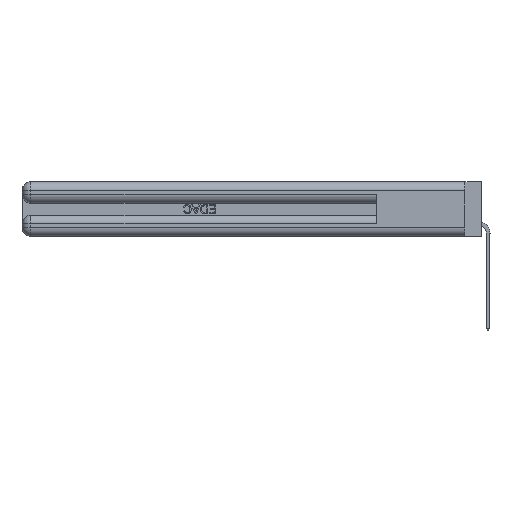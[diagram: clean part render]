
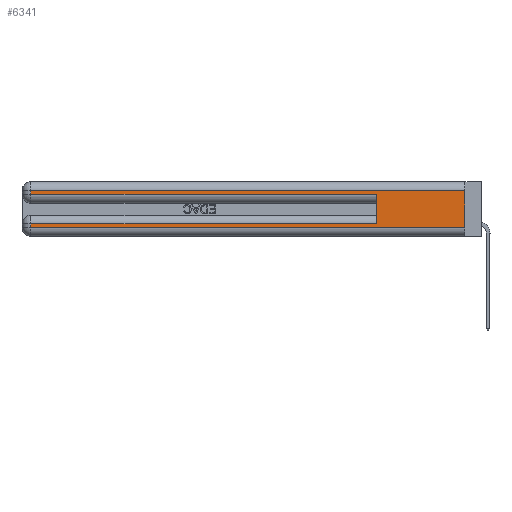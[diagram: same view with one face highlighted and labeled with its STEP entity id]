
A CAD part, left-side view. The second image highlights one B-rep face of the part: STEP entity #6341.
In plain terms, the highlighted planar face has unit normal (-1, 0, 0).
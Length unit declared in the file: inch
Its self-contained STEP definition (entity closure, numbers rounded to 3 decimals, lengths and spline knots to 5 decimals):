
#353 = VECTOR ( 'NONE', #24202, 39.37008 ) ;
#382 = CARTESIAN_POINT ( 'NONE',  ( 0., 0., 0.06 ) ) ;
#565 = EDGE_CURVE ( 'NONE', #36452, #20601, #5713, .T. ) ;
#597 = VECTOR ( 'NONE', #34146, 39.37008 ) ;
#1828 = VERTEX_POINT ( 'NONE', #7618 ) ;
#2345 = CARTESIAN_POINT ( 'NONE',  ( 0., 2.94, 0.37 ) ) ;
#2693 = LINE ( 'NONE', #42257, #31946 ) ;
#2855 = ORIENTED_EDGE ( 'NONE', *, *, #39296, .T. ) ;
#3365 = LINE ( 'NONE', #9745, #29415 ) ;
#3760 = CARTESIAN_POINT ( 'NONE',  ( 0., 2.94, 0.085 ) ) ;
#4525 = EDGE_CURVE ( 'NONE', #1828, #20601, #2693, .T. ) ;
#5074 = CARTESIAN_POINT ( 'NONE',  ( 0., 2.94, 0.31 ) ) ;
#5713 = LINE ( 'NONE', #382, #32272 ) ;
#5806 = VECTOR ( 'NONE', #27637, 39.37008 ) ;
#6089 = ORIENTED_EDGE ( 'NONE', *, *, #41790, .T. ) ;
#6341 = ADVANCED_FACE ( 'NONE', ( #25330 ), #29210, .F. ) ;
#6717 = LINE ( 'NONE', #9881, #597 ) ;
#7503 = ORIENTED_EDGE ( 'NONE', *, *, #22919, .T. ) ;
#7618 = CARTESIAN_POINT ( 'NONE',  ( 0., 0., 0.31 ) ) ;
#8039 = LINE ( 'NONE', #34278, #353 ) ;
#9089 = DIRECTION ( 'NONE',  ( 0., 0., -1. ) ) ;
#9263 = CARTESIAN_POINT ( 'NONE',  ( 0., 0., 0.37 ) ) ;
#9745 = CARTESIAN_POINT ( 'NONE',  ( 0., 0., 0.285 ) ) ;
#9881 = CARTESIAN_POINT ( 'NONE',  ( 0., 0., 0.31 ) ) ;
#11447 = CARTESIAN_POINT ( 'NONE',  ( 0., 2.94, 0.285 ) ) ;
#12366 = ORIENTED_EDGE ( 'NONE', *, *, #565, .T. ) ;
#12652 = VERTEX_POINT ( 'NONE', #11447 ) ;
#13560 = CARTESIAN_POINT ( 'NONE',  ( 0., 0.6, 0.085 ) ) ;
#15887 = DIRECTION ( 'NONE',  ( 0., 0., -1. ) ) ;
#19194 = DIRECTION ( 'NONE',  ( 0., 0., 1. ) ) ;
#19713 = DIRECTION ( 'NONE',  ( 0., -1., 0. ) ) ;
#20581 = ORIENTED_EDGE ( 'NONE', *, *, #20896, .T. ) ;
#20601 = VERTEX_POINT ( 'NONE', #23015 ) ;
#20896 = EDGE_CURVE ( 'NONE', #20955, #40699, #30249, .T. ) ;
#20955 = VERTEX_POINT ( 'NONE', #13560 ) ;
#20996 = ORIENTED_EDGE ( 'NONE', *, *, #39722, .F. ) ;
#21216 = LINE ( 'NONE', #43363, #38625 ) ;
#22732 = DIRECTION ( 'NONE',  ( 0., -1., 0. ) ) ;
#22919 = EDGE_CURVE ( 'NONE', #1828, #26209, #6717, .T. ) ;
#23015 = CARTESIAN_POINT ( 'NONE',  ( 0., 0., 0.06 ) ) ;
#23701 = CARTESIAN_POINT ( 'NONE',  ( 0., 0., 0.085 ) ) ;
#24202 = DIRECTION ( 'NONE',  ( 0., 0., -1. ) ) ;
#24975 = ORIENTED_EDGE ( 'NONE', *, *, #44619, .T. ) ;
#25330 = FACE_OUTER_BOUND ( 'NONE', #37698, .T. ) ;
#26209 = VERTEX_POINT ( 'NONE', #5074 ) ;
#27637 = DIRECTION ( 'NONE',  ( 0., 1., 0. ) ) ;
#29210 = PLANE ( 'NONE',  #44918 ) ;
#29415 = VECTOR ( 'NONE', #19713, 39.37008 ) ;
#30249 = LINE ( 'NONE', #23701, #5806 ) ;
#30815 = CARTESIAN_POINT ( 'NONE',  ( 0., 2.94, 0.06 ) ) ;
#31375 = VECTOR ( 'NONE', #9089, 39.37008 ) ;
#31946 = VECTOR ( 'NONE', #35738, 39.37008 ) ;
#32272 = VECTOR ( 'NONE', #22732, 39.37008 ) ;
#33648 = DIRECTION ( 'NONE',  ( 1., 0., 0. ) ) ;
#33723 = VERTEX_POINT ( 'NONE', #40663 ) ;
#34146 = DIRECTION ( 'NONE',  ( 0., 1., 0. ) ) ;
#34278 = CARTESIAN_POINT ( 'NONE',  ( 0., 2.94, 0.37 ) ) ;
#35738 = DIRECTION ( 'NONE',  ( 0., 0., -1. ) ) ;
#36452 = VERTEX_POINT ( 'NONE', #30815 ) ;
#37698 = EDGE_LOOP ( 'NONE', ( #44507, #7503, #6089, #2855, #20996, #20581, #24975, #12366 ) ) ;
#37970 = LINE ( 'NONE', #2345, #31375 ) ;
#38625 = VECTOR ( 'NONE', #19194, 39.37008 ) ;
#39296 = EDGE_CURVE ( 'NONE', #12652, #33723, #3365, .T. ) ;
#39722 = EDGE_CURVE ( 'NONE', #20955, #33723, #21216, .T. ) ;
#40663 = CARTESIAN_POINT ( 'NONE',  ( 0., 0.6, 0.285 ) ) ;
#40699 = VERTEX_POINT ( 'NONE', #3760 ) ;
#41790 = EDGE_CURVE ( 'NONE', #26209, #12652, #8039, .T. ) ;
#42257 = CARTESIAN_POINT ( 'NONE',  ( 0., 0., 0.37 ) ) ;
#43363 = CARTESIAN_POINT ( 'NONE',  ( 0., 0.6, 0.145 ) ) ;
#44507 = ORIENTED_EDGE ( 'NONE', *, *, #4525, .F. ) ;
#44619 = EDGE_CURVE ( 'NONE', #40699, #36452, #37970, .T. ) ;
#44918 = AXIS2_PLACEMENT_3D ( 'NONE', #9263, #33648, #15887 ) ;
